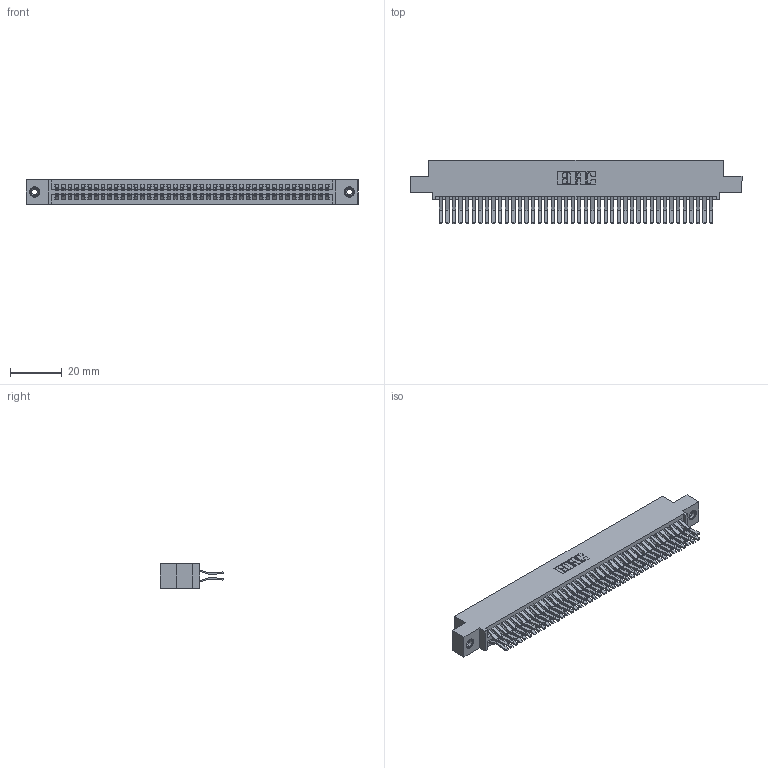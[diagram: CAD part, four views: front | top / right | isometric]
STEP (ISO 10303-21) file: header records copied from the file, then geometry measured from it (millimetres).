
FILE_DESCRIPTION (( 'STEP AP203' ), '1' );
FILE_NAME ('395-084-560-508.STEP', '2019-10-25T10:45:21', ( '' ), ( '' ), 'SwSTEP 2.0', 'SolidWorks 2016', '' );
FILE_SCHEMA (( 'CONFIG_CONTROL_DESIGN' ));
Length unit declared in the file: inch
Products named in the file (4): 345 Part_0.110 Offset - 0.156 Dia-TI; 345-292-001_560 Tail; 345-250-001_345-250-003-102; 395-084-560-508
Assembly tree (87 placements, depth 2):
  395-084-560-508
    345 Part_0.110 Offset - 0.156 Dia-TI
    345-292-001_560 Tail  x84
    345-250-001_345-250-003-102  x2
Bounding box: 127.89 x 24.45 x 9.4 mm (x, y, z)
Volume: 12894 mm3; surface area: 20581.8 mm2
Topology: 87 solids, 87 shells, 4558 faces, 13509 edges, 8886 vertices
Faces by surface type: plane 2888, cylinder 1654, cone 12, torus 4
Entity records: 34360 total; most frequent: CARTESIAN_POINT 5743, ORIENTED_EDGE 5670, DIRECTION 5093, EDGE_CURVE 2835, VECTOR 2511, LINE 2511, VERTEX_POINT 1884, AXIS2_PLACEMENT_3D 1291
